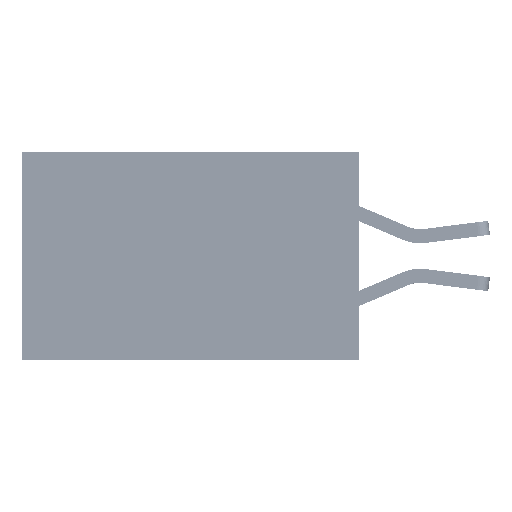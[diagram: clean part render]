
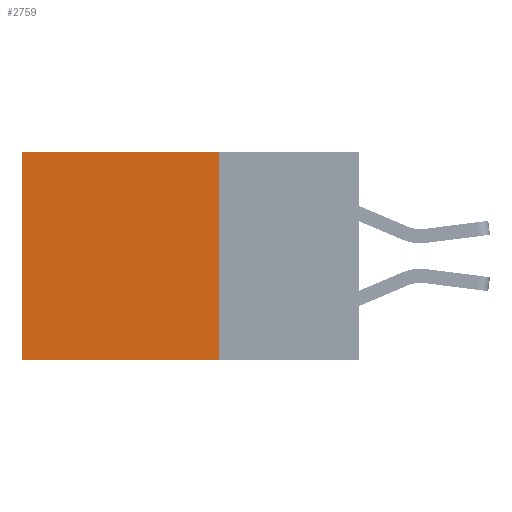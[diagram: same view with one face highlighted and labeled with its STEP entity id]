
A CAD part, left-side view. The second image highlights one B-rep face of the part: STEP entity #2759.
In plain terms, the highlighted planar face has unit normal (-1, 0, 0).
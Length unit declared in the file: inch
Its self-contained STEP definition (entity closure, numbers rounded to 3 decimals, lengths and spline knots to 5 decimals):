
#261 = ORIENTED_EDGE ( 'NONE', *, *, #2842, .F. ) ;
#1770 = LINE ( 'NONE', #29387, #17410 ) ;
#2759 = ADVANCED_FACE ( 'NONE', ( #14468 ), #28431, .F. ) ;
#2840 = DIRECTION ( 'NONE',  ( 0., 1., 0. ) ) ;
#2842 = EDGE_CURVE ( 'NONE', #5328, #33622, #1770, .T. ) ;
#4145 = EDGE_CURVE ( 'NONE', #5328, #14482, #21444, .T. ) ;
#4188 = CARTESIAN_POINT ( 'NONE',  ( 0.2875, 0.25, 0. ) ) ;
#4887 = DIRECTION ( 'NONE',  ( 1., 0., 0. ) ) ;
#5328 = VERTEX_POINT ( 'NONE', #4188 ) ;
#5383 = ORIENTED_EDGE ( 'NONE', *, *, #4145, .T. ) ;
#5389 = DIRECTION ( 'NONE',  ( 0., 0., -1. ) ) ;
#5798 = AXIS2_PLACEMENT_3D ( 'NONE', #28070, #4887, #5389 ) ;
#6224 = CARTESIAN_POINT ( 'NONE',  ( 0.2875, 0.25, -0.37 ) ) ;
#8253 = LINE ( 'NONE', #12568, #34751 ) ;
#9970 = CARTESIAN_POINT ( 'NONE',  ( 0.2875, 0.25, -0.37 ) ) ;
#11499 = DIRECTION ( 'NONE',  ( 0., 0., -1. ) ) ;
#12568 = CARTESIAN_POINT ( 'NONE',  ( 0.2875, 0.6, 0. ) ) ;
#14468 = FACE_OUTER_BOUND ( 'NONE', #35438, .T. ) ;
#14482 = VERTEX_POINT ( 'NONE', #31385 ) ;
#14681 = EDGE_CURVE ( 'NONE', #14482, #31844, #8253, .T. ) ;
#15003 = DIRECTION ( 'NONE',  ( 0., 0., -1. ) ) ;
#17410 = VECTOR ( 'NONE', #15003, 39.37008 ) ;
#21444 = LINE ( 'NONE', #27113, #29962 ) ;
#24996 = VECTOR ( 'NONE', #2840, 39.37008 ) ;
#26318 = LINE ( 'NONE', #6224, #24996 ) ;
#27113 = CARTESIAN_POINT ( 'NONE',  ( 0.2875, 0.25, 0. ) ) ;
#27908 = EDGE_CURVE ( 'NONE', #33622, #31844, #26318, .T. ) ;
#28070 = CARTESIAN_POINT ( 'NONE',  ( 0.2875, 0.25, 0. ) ) ;
#28431 = PLANE ( 'NONE',  #5798 ) ;
#29387 = CARTESIAN_POINT ( 'NONE',  ( 0.2875, 0.25, 0. ) ) ;
#29962 = VECTOR ( 'NONE', #29982, 39.37008 ) ;
#29982 = DIRECTION ( 'NONE',  ( 0., 1., 0. ) ) ;
#31385 = CARTESIAN_POINT ( 'NONE',  ( 0.2875, 0.6, 0. ) ) ;
#31844 = VERTEX_POINT ( 'NONE', #34279 ) ;
#33321 = ORIENTED_EDGE ( 'NONE', *, *, #14681, .T. ) ;
#33622 = VERTEX_POINT ( 'NONE', #9970 ) ;
#34279 = CARTESIAN_POINT ( 'NONE',  ( 0.2875, 0.6, -0.37 ) ) ;
#34751 = VECTOR ( 'NONE', #11499, 39.37008 ) ;
#35438 = EDGE_LOOP ( 'NONE', ( #33321, #36788, #261, #5383 ) ) ;
#36788 = ORIENTED_EDGE ( 'NONE', *, *, #27908, .F. ) ;
